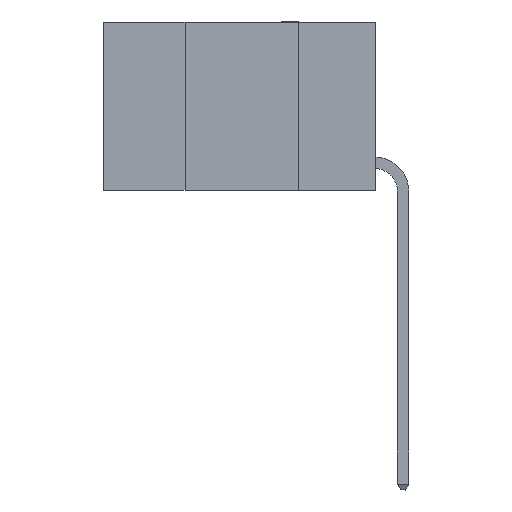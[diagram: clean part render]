
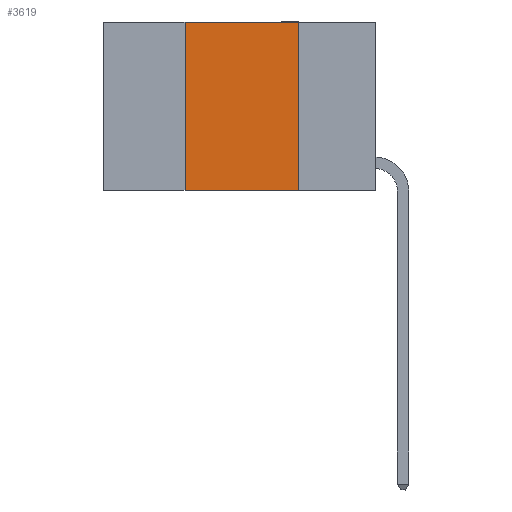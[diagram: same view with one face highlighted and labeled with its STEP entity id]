
A CAD part, left-side view. The second image highlights one B-rep face of the part: STEP entity #3619.
In plain terms, the highlighted planar face has unit normal (-1, 0, 0).
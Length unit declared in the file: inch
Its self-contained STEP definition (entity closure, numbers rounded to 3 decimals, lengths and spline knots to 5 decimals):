
#222 = VECTOR ( 'NONE', #7562, 39.37008 ) ;
#756 = FACE_OUTER_BOUND ( 'NONE', #1702, .T. ) ;
#1151 = VECTOR ( 'NONE', #7516, 39.37008 ) ;
#1195 = VERTEX_POINT ( 'NONE', #7151 ) ;
#1278 = CARTESIAN_POINT ( 'NONE',  ( 0., 0.17, -0.37 ) ) ;
#1387 = CARTESIAN_POINT ( 'NONE',  ( 0., 0.6, -0.37 ) ) ;
#1702 = EDGE_LOOP ( 'NONE', ( #2624, #5859, #7810, #5827 ) ) ;
#1776 = LINE ( 'NONE', #2199, #5353 ) ;
#2199 = CARTESIAN_POINT ( 'NONE',  ( 0., 0.17, 0. ) ) ;
#2222 = LINE ( 'NONE', #1387, #222 ) ;
#2236 = CARTESIAN_POINT ( 'NONE',  ( 0., 0.17, 0. ) ) ;
#2624 = ORIENTED_EDGE ( 'NONE', *, *, #7792, .F. ) ;
#2803 = EDGE_CURVE ( 'NONE', #6751, #1195, #8345, .T. ) ;
#2882 = DIRECTION ( 'NONE',  ( 0., 0., -1. ) ) ;
#2948 = DIRECTION ( 'NONE',  ( 0., 0., -1. ) ) ;
#3019 = VERTEX_POINT ( 'NONE', #1278 ) ;
#3464 = CARTESIAN_POINT ( 'NONE',  ( 0., 0.42, -0.37 ) ) ;
#3516 = EDGE_CURVE ( 'NONE', #1195, #6048, #6817, .T. ) ;
#3619 = ADVANCED_FACE ( 'NONE', ( #756 ), #8707, .F. ) ;
#5094 = VECTOR ( 'NONE', #8056, 39.37008 ) ;
#5353 = VECTOR ( 'NONE', #2948, 39.37008 ) ;
#5395 = CARTESIAN_POINT ( 'NONE',  ( 0., 0.42, 0. ) ) ;
#5529 = CARTESIAN_POINT ( 'NONE',  ( 0., 0.6, 0. ) ) ;
#5827 = ORIENTED_EDGE ( 'NONE', *, *, #8759, .T. ) ;
#5859 = ORIENTED_EDGE ( 'NONE', *, *, #3516, .F. ) ;
#6048 = VERTEX_POINT ( 'NONE', #2236 ) ;
#6751 = VERTEX_POINT ( 'NONE', #3464 ) ;
#6817 = LINE ( 'NONE', #5529, #5094 ) ;
#6913 = CARTESIAN_POINT ( 'NONE',  ( 0., 0.6, 0. ) ) ;
#6938 = DIRECTION ( 'NONE',  ( 1., 0., 0. ) ) ;
#7151 = CARTESIAN_POINT ( 'NONE',  ( 0., 0.42, 0. ) ) ;
#7516 = DIRECTION ( 'NONE',  ( 0., 0., 1. ) ) ;
#7562 = DIRECTION ( 'NONE',  ( 0., -1., 0. ) ) ;
#7752 = AXIS2_PLACEMENT_3D ( 'NONE', #6913, #6938, #2882 ) ;
#7792 = EDGE_CURVE ( 'NONE', #6048, #3019, #1776, .T. ) ;
#7810 = ORIENTED_EDGE ( 'NONE', *, *, #2803, .F. ) ;
#8056 = DIRECTION ( 'NONE',  ( 0., -1., 0. ) ) ;
#8345 = LINE ( 'NONE', #5395, #1151 ) ;
#8707 = PLANE ( 'NONE',  #7752 ) ;
#8759 = EDGE_CURVE ( 'NONE', #6751, #3019, #2222, .T. ) ;
